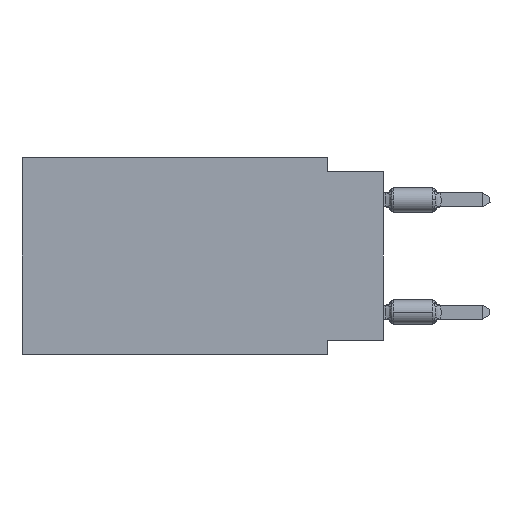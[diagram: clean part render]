
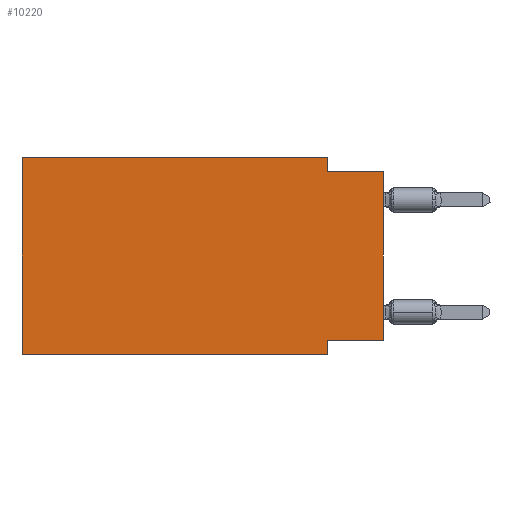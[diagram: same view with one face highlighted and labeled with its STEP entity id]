
A CAD part, left-side view. The second image highlights one B-rep face of the part: STEP entity #10220.
In plain terms, the highlighted planar face has unit normal (-1, 0, 0).
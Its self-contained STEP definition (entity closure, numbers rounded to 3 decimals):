
#1861 = CARTESIAN_POINT ( 'NONE',  ( 0., 16.383, 0. ) ) ;
#1947 = VERTEX_POINT ( 'NONE', #22881 ) ;
#2437 = CARTESIAN_POINT ( 'NONE',  ( 0., 2.54, -0.635 ) ) ;
#4610 = VECTOR ( 'NONE', #30547, 1000. ) ;
#4941 = EDGE_CURVE ( 'NONE', #37395, #53245, #17224, .T. ) ;
#6043 = EDGE_CURVE ( 'NONE', #34862, #53245, #38968, .T. ) ;
#6964 = VECTOR ( 'NONE', #9442, 1000. ) ;
#8092 = ORIENTED_EDGE ( 'NONE', *, *, #25545, .F. ) ;
#8331 = DIRECTION ( 'NONE',  ( 0., 0., -1. ) ) ;
#8774 = DIRECTION ( 'NONE',  ( 0., 0., -1. ) ) ;
#9442 = DIRECTION ( 'NONE',  ( 0., 0., -1. ) ) ;
#10056 = CARTESIAN_POINT ( 'NONE',  ( 0., 2.54, -8.255 ) ) ;
#10101 = LINE ( 'NONE', #39637, #6964 ) ;
#10115 = CARTESIAN_POINT ( 'NONE',  ( 0., 0., -0.635 ) ) ;
#10220 = ADVANCED_FACE ( 'NONE', ( #56754 ), #42760, .F. ) ;
#12853 = CARTESIAN_POINT ( 'NONE',  ( 0., 16.383, 0. ) ) ;
#14529 = ORIENTED_EDGE ( 'NONE', *, *, #15349, .F. ) ;
#15349 = EDGE_CURVE ( 'NONE', #37395, #48161, #47916, .T. ) ;
#16161 = EDGE_CURVE ( 'NONE', #1947, #34862, #62368, .T. ) ;
#17224 = LINE ( 'NONE', #51944, #38286 ) ;
#19036 = CARTESIAN_POINT ( 'NONE',  ( 0., 16.383, -8.89 ) ) ;
#19729 = ORIENTED_EDGE ( 'NONE', *, *, #16161, .F. ) ;
#19930 = ORIENTED_EDGE ( 'NONE', *, *, #6043, .F. ) ;
#22764 = VERTEX_POINT ( 'NONE', #52197 ) ;
#22881 = CARTESIAN_POINT ( 'NONE',  ( 0., 0., -8.255 ) ) ;
#23225 = DIRECTION ( 'NONE',  ( 0., 0., 1. ) ) ;
#23297 = ORIENTED_EDGE ( 'NONE', *, *, #60057, .T. ) ;
#25545 = EDGE_CURVE ( 'NONE', #22764, #62699, #10101, .T. ) ;
#27584 = EDGE_CURVE ( 'NONE', #62699, #32206, #55245, .T. ) ;
#28340 = VECTOR ( 'NONE', #23225, 1000. ) ;
#30547 = DIRECTION ( 'NONE',  ( 0., -1., 0. ) ) ;
#31732 = ORIENTED_EDGE ( 'NONE', *, *, #27584, .F. ) ;
#31751 = CARTESIAN_POINT ( 'NONE',  ( 0., 0., 0. ) ) ;
#32206 = VERTEX_POINT ( 'NONE', #54105 ) ;
#32893 = VECTOR ( 'NONE', #8774, 1000. ) ;
#32982 = DIRECTION ( 'NONE',  ( 0., -1., 0. ) ) ;
#33011 = CARTESIAN_POINT ( 'NONE',  ( 0., 16.383, 0. ) ) ;
#34862 = VERTEX_POINT ( 'NONE', #10056 ) ;
#36720 = CARTESIAN_POINT ( 'NONE',  ( 0., 0., -8.255 ) ) ;
#37395 = VERTEX_POINT ( 'NONE', #19036 ) ;
#38286 = VECTOR ( 'NONE', #62324, 1000. ) ;
#38968 = LINE ( 'NONE', #63312, #32893 ) ;
#39637 = CARTESIAN_POINT ( 'NONE',  ( 0., 2.54, 0. ) ) ;
#39903 = ORIENTED_EDGE ( 'NONE', *, *, #4941, .T. ) ;
#41358 = CARTESIAN_POINT ( 'NONE',  ( 0., 16.383, 0. ) ) ;
#41450 = VECTOR ( 'NONE', #32982, 1000. ) ;
#42760 = PLANE ( 'NONE',  #48352 ) ;
#42903 = EDGE_LOOP ( 'NONE', ( #23297, #31732, #8092, #63905, #14529, #39903, #19930, #19729 ) ) ;
#45775 = CARTESIAN_POINT ( 'NONE',  ( 0., 2.54, -8.89 ) ) ;
#46054 = DIRECTION ( 'NONE',  ( 0., 0., 1. ) ) ;
#46345 = LINE ( 'NONE', #1861, #41450 ) ;
#47916 = LINE ( 'NONE', #12853, #28340 ) ;
#48161 = VERTEX_POINT ( 'NONE', #41358 ) ;
#48352 = AXIS2_PLACEMENT_3D ( 'NONE', #33011, #52830, #8331 ) ;
#51944 = CARTESIAN_POINT ( 'NONE',  ( 0., 16.383, -8.89 ) ) ;
#51982 = DIRECTION ( 'NONE',  ( 0., 1., 0. ) ) ;
#52197 = CARTESIAN_POINT ( 'NONE',  ( 0., 2.54, 0. ) ) ;
#52203 = LINE ( 'NONE', #31751, #63696 ) ;
#52663 = EDGE_CURVE ( 'NONE', #48161, #22764, #46345, .T. ) ;
#52830 = DIRECTION ( 'NONE',  ( 1., 0., 0. ) ) ;
#53245 = VERTEX_POINT ( 'NONE', #45775 ) ;
#54105 = CARTESIAN_POINT ( 'NONE',  ( 0., 0., -0.635 ) ) ;
#55245 = LINE ( 'NONE', #10115, #4610 ) ;
#56754 = FACE_OUTER_BOUND ( 'NONE', #42903, .T. ) ;
#60057 = EDGE_CURVE ( 'NONE', #1947, #32206, #52203, .T. ) ;
#60565 = VECTOR ( 'NONE', #51982, 1000. ) ;
#62324 = DIRECTION ( 'NONE',  ( 0., -1., 0. ) ) ;
#62368 = LINE ( 'NONE', #36720, #60565 ) ;
#62699 = VERTEX_POINT ( 'NONE', #2437 ) ;
#63312 = CARTESIAN_POINT ( 'NONE',  ( 0., 2.54, -8.89 ) ) ;
#63696 = VECTOR ( 'NONE', #46054, 1000. ) ;
#63905 = ORIENTED_EDGE ( 'NONE', *, *, #52663, .F. ) ;
